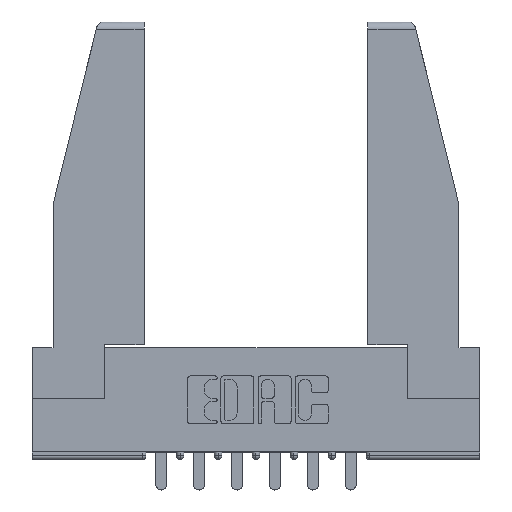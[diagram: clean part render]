
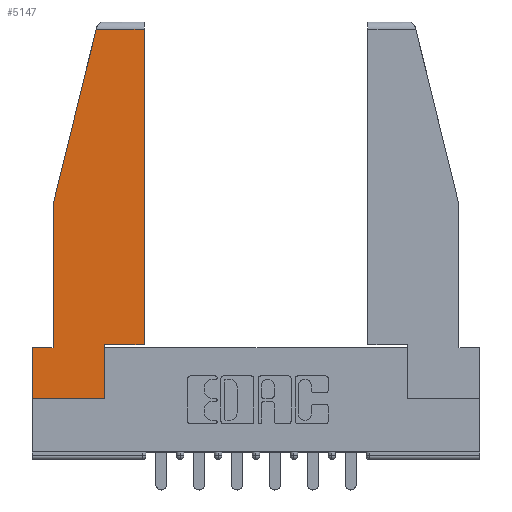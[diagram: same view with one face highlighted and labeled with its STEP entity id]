
A CAD part, top view. The second image highlights one B-rep face of the part: STEP entity #5147.
In plain terms, the highlighted planar face has unit normal (0, 0, 1).
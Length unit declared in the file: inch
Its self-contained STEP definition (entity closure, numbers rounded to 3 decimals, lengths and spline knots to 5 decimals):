
#134 = DIRECTION ( 'NONE',  ( 1., 0., 0. ) ) ;
#152 = VERTEX_POINT ( 'NONE', #3132 ) ;
#178 = LINE ( 'NONE', #9243, #6732 ) ;
#197 = CARTESIAN_POINT ( 'NONE',  ( 0.086, 0.8, 0. ) ) ;
#228 = ORIENTED_EDGE ( 'NONE', *, *, #6411, .T. ) ;
#276 = LINE ( 'NONE', #4827, #8093 ) ;
#682 = ORIENTED_EDGE ( 'NONE', *, *, #10972, .T. ) ;
#795 = CARTESIAN_POINT ( 'NONE',  ( 0.271, 1.55, 0. ) ) ;
#916 = ORIENTED_EDGE ( 'NONE', *, *, #10219, .T. ) ;
#926 = EDGE_LOOP ( 'NONE', ( #12928, #228, #10552, #2108, #4158, #6200, #682, #3455, #916 ) ) ;
#1289 = VECTOR ( 'NONE', #6939, 39.37008 ) ;
#2026 = EDGE_CURVE ( 'NONE', #7692, #7907, #276, .T. ) ;
#2108 = ORIENTED_EDGE ( 'NONE', *, *, #4831, .T. ) ;
#2129 = DIRECTION ( 'NONE',  ( 1., 0., 0. ) ) ;
#2250 = DIRECTION ( 'NONE',  ( 0., -1., 0. ) ) ;
#2546 = VECTOR ( 'NONE', #8017, 39.37008 ) ;
#2604 = EDGE_CURVE ( 'NONE', #9582, #7692, #12090, .T. ) ;
#2775 = VECTOR ( 'NONE', #9413, 39.37008 ) ;
#3132 = CARTESIAN_POINT ( 'NONE',  ( 0.461, 1.52, 0. ) ) ;
#3455 = ORIENTED_EDGE ( 'NONE', *, *, #12697, .T. ) ;
#4130 = CARTESIAN_POINT ( 'NONE',  ( 0., 0., 0. ) ) ;
#4158 = ORIENTED_EDGE ( 'NONE', *, *, #2604, .T. ) ;
#4247 = VECTOR ( 'NONE', #7045, 39.37008 ) ;
#4316 = VERTEX_POINT ( 'NONE', #11114 ) ;
#4422 = EDGE_CURVE ( 'NONE', #10494, #152, #10129, .T. ) ;
#4647 = LINE ( 'NONE', #10357, #6740 ) ;
#4827 = CARTESIAN_POINT ( 'NONE',  ( 0., 0.21, 0. ) ) ;
#4831 = EDGE_CURVE ( 'NONE', #12790, #9582, #11238, .T. ) ;
#5147 = ADVANCED_FACE ( 'NONE', ( #9942 ), #8172, .T. ) ;
#5362 = CARTESIAN_POINT ( 'NONE',  ( 0.461, 0.223, 0. ) ) ;
#5505 = CARTESIAN_POINT ( 'NONE',  ( 0., 1.52, 0. ) ) ;
#5552 = DIRECTION ( 'NONE',  ( 1., 0., 0. ) ) ;
#5950 = EDGE_CURVE ( 'NONE', #6551, #12790, #11041, .T. ) ;
#5985 = DIRECTION ( 'NONE',  ( 0., -1., 0. ) ) ;
#6200 = ORIENTED_EDGE ( 'NONE', *, *, #2026, .T. ) ;
#6326 = CARTESIAN_POINT ( 'NONE',  ( 0.461, 0.223, 0. ) ) ;
#6411 = EDGE_CURVE ( 'NONE', #152, #6551, #8612, .T. ) ;
#6551 = VERTEX_POINT ( 'NONE', #10822 ) ;
#6732 = VECTOR ( 'NONE', #134, 39.37008 ) ;
#6740 = VECTOR ( 'NONE', #2129, 39.37008 ) ;
#6939 = DIRECTION ( 'NONE',  ( -0.239, -0.971, 0. ) ) ;
#7045 = DIRECTION ( 'NONE',  ( -1., 0., 0. ) ) ;
#7333 = LINE ( 'NONE', #10001, #2546 ) ;
#7692 = VERTEX_POINT ( 'NONE', #9918 ) ;
#7824 = VECTOR ( 'NONE', #8437, 39.37008 ) ;
#7907 = VERTEX_POINT ( 'NONE', #9114 ) ;
#8011 = CARTESIAN_POINT ( 'NONE',  ( 0.086, 0.21, 0. ) ) ;
#8017 = DIRECTION ( 'NONE',  ( 0., 1., 0. ) ) ;
#8093 = VECTOR ( 'NONE', #5985, 39.37008 ) ;
#8172 = PLANE ( 'NONE',  #12233 ) ;
#8437 = DIRECTION ( 'NONE',  ( -1., 0., 0. ) ) ;
#8496 = VECTOR ( 'NONE', #2250, 39.37008 ) ;
#8612 = LINE ( 'NONE', #5505, #7824 ) ;
#8956 = CARTESIAN_POINT ( 'NONE',  ( 0., 0.21, 0. ) ) ;
#9114 = CARTESIAN_POINT ( 'NONE',  ( 0., 0., 0. ) ) ;
#9243 = CARTESIAN_POINT ( 'NONE',  ( 0., 0., 0. ) ) ;
#9374 = CARTESIAN_POINT ( 'NONE',  ( 0.086, 0.8, 0. ) ) ;
#9413 = DIRECTION ( 'NONE',  ( 0., 1., 0. ) ) ;
#9582 = VERTEX_POINT ( 'NONE', #8011 ) ;
#9918 = CARTESIAN_POINT ( 'NONE',  ( 0., 0.21, 0. ) ) ;
#9942 = FACE_OUTER_BOUND ( 'NONE', #926, .T. ) ;
#10001 = CARTESIAN_POINT ( 'NONE',  ( 0.297, 0., 0. ) ) ;
#10129 = LINE ( 'NONE', #6326, #2775 ) ;
#10219 = EDGE_CURVE ( 'NONE', #4316, #10494, #4647, .T. ) ;
#10357 = CARTESIAN_POINT ( 'NONE',  ( 0.297, 0.223, 0. ) ) ;
#10494 = VERTEX_POINT ( 'NONE', #5362 ) ;
#10552 = ORIENTED_EDGE ( 'NONE', *, *, #5950, .T. ) ;
#10822 = CARTESIAN_POINT ( 'NONE',  ( 0.2636, 1.52, 0. ) ) ;
#10972 = EDGE_CURVE ( 'NONE', #7907, #12692, #178, .T. ) ;
#11041 = LINE ( 'NONE', #795, #1289 ) ;
#11114 = CARTESIAN_POINT ( 'NONE',  ( 0.297, 0.223, 0. ) ) ;
#11238 = LINE ( 'NONE', #197, #8496 ) ;
#11727 = DIRECTION ( 'NONE',  ( 0., 0., 1. ) ) ;
#12090 = LINE ( 'NONE', #8956, #4247 ) ;
#12233 = AXIS2_PLACEMENT_3D ( 'NONE', #4130, #11727, #5552 ) ;
#12692 = VERTEX_POINT ( 'NONE', #13089 ) ;
#12697 = EDGE_CURVE ( 'NONE', #12692, #4316, #7333, .T. ) ;
#12790 = VERTEX_POINT ( 'NONE', #9374 ) ;
#12928 = ORIENTED_EDGE ( 'NONE', *, *, #4422, .T. ) ;
#13089 = CARTESIAN_POINT ( 'NONE',  ( 0.297, 0., 0. ) ) ;
